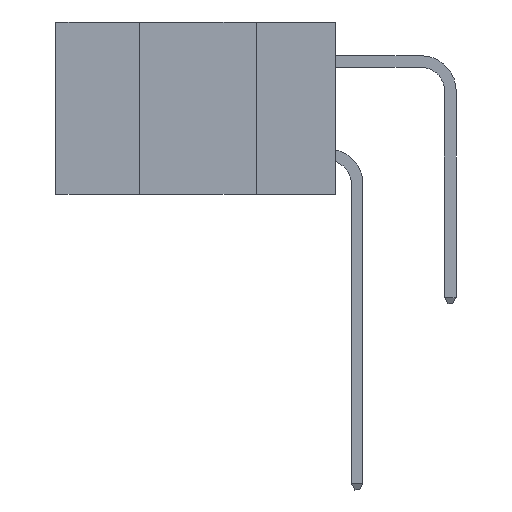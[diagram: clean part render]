
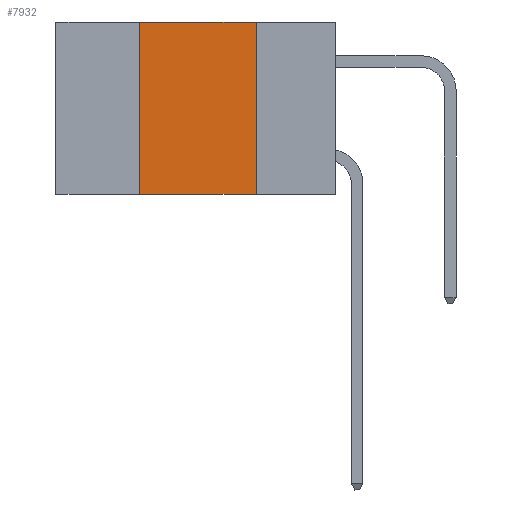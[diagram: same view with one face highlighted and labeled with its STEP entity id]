
A CAD part, left-side view. The second image highlights one B-rep face of the part: STEP entity #7932.
In plain terms, the highlighted planar face has unit normal (-1, 0, 0).
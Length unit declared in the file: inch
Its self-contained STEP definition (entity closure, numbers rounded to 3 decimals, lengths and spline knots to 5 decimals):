
#104 = FACE_OUTER_BOUND ( 'NONE', #2291, .T. ) ;
#153 = LINE ( 'NONE', #10878, #4950 ) ;
#193 = EDGE_CURVE ( 'NONE', #11217, #9031, #2081, .T. ) ;
#1456 = ORIENTED_EDGE ( 'NONE', *, *, #1535, .F. ) ;
#1535 = EDGE_CURVE ( 'NONE', #9031, #3601, #11531, .T. ) ;
#1676 = DIRECTION ( 'NONE',  ( 0., -1., 0. ) ) ;
#1712 = LINE ( 'NONE', #8386, #7026 ) ;
#2081 = LINE ( 'NONE', #9117, #11563 ) ;
#2291 = EDGE_LOOP ( 'NONE', ( #1456, #11268, #9487, #11837 ) ) ;
#2875 = CARTESIAN_POINT ( 'NONE',  ( 0., 0.42, -0.37 ) ) ;
#3196 = DIRECTION ( 'NONE',  ( 0., -1., 0. ) ) ;
#3601 = VERTEX_POINT ( 'NONE', #9019 ) ;
#3918 = PLANE ( 'NONE',  #9033 ) ;
#4950 = VECTOR ( 'NONE', #1676, 39.37008 ) ;
#5011 = EDGE_CURVE ( 'NONE', #8998, #11217, #1712, .T. ) ;
#5823 = DIRECTION ( 'NONE',  ( 0., 0., -1. ) ) ;
#6740 = VECTOR ( 'NONE', #7237, 39.37008 ) ;
#7026 = VECTOR ( 'NONE', #8347, 39.37008 ) ;
#7237 = DIRECTION ( 'NONE',  ( 0., 0., -1. ) ) ;
#7932 = ADVANCED_FACE ( 'NONE', ( #104 ), #3918, .F. ) ;
#8347 = DIRECTION ( 'NONE',  ( 0., 0., 1. ) ) ;
#8386 = CARTESIAN_POINT ( 'NONE',  ( 0., 0.42, 0. ) ) ;
#8807 = CARTESIAN_POINT ( 'NONE',  ( 0., 0.17, 0. ) ) ;
#8998 = VERTEX_POINT ( 'NONE', #2875 ) ;
#9019 = CARTESIAN_POINT ( 'NONE',  ( 0., 0.17, -0.37 ) ) ;
#9031 = VERTEX_POINT ( 'NONE', #9441 ) ;
#9033 = AXIS2_PLACEMENT_3D ( 'NONE', #10334, #11234, #5823 ) ;
#9117 = CARTESIAN_POINT ( 'NONE',  ( 0., 0.6, 0. ) ) ;
#9441 = CARTESIAN_POINT ( 'NONE',  ( 0., 0.17, 0. ) ) ;
#9487 = ORIENTED_EDGE ( 'NONE', *, *, #5011, .F. ) ;
#10334 = CARTESIAN_POINT ( 'NONE',  ( 0., 0.6, 0. ) ) ;
#10766 = CARTESIAN_POINT ( 'NONE',  ( 0., 0.42, 0. ) ) ;
#10878 = CARTESIAN_POINT ( 'NONE',  ( 0., 0.6, -0.37 ) ) ;
#11217 = VERTEX_POINT ( 'NONE', #10766 ) ;
#11234 = DIRECTION ( 'NONE',  ( 1., 0., 0. ) ) ;
#11268 = ORIENTED_EDGE ( 'NONE', *, *, #193, .F. ) ;
#11327 = EDGE_CURVE ( 'NONE', #8998, #3601, #153, .T. ) ;
#11531 = LINE ( 'NONE', #8807, #6740 ) ;
#11563 = VECTOR ( 'NONE', #3196, 39.37008 ) ;
#11837 = ORIENTED_EDGE ( 'NONE', *, *, #11327, .T. ) ;
